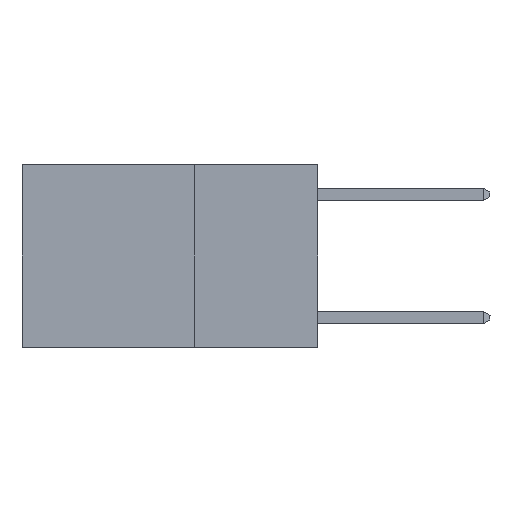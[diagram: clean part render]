
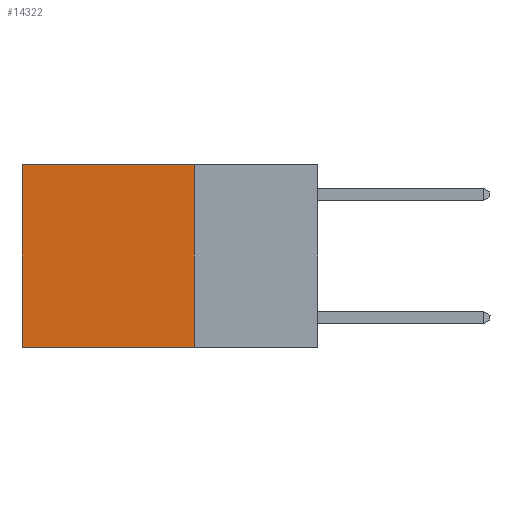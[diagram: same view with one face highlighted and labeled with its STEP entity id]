
A CAD part, left-side view. The second image highlights one B-rep face of the part: STEP entity #14322.
In plain terms, the highlighted planar face has unit normal (-1, 0, 0).
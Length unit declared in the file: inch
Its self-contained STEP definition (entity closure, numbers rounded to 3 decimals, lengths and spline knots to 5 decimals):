
#82 = PLANE ( 'NONE',  #14268 ) ;
#537 = LINE ( 'NONE', #14265, #15132 ) ;
#1487 = FACE_OUTER_BOUND ( 'NONE', #11805, .T. ) ;
#1881 = VERTEX_POINT ( 'NONE', #3082 ) ;
#2308 = VECTOR ( 'NONE', #5954, 39.37008 ) ;
#2724 = ORIENTED_EDGE ( 'NONE', *, *, #12147, .T. ) ;
#3082 = CARTESIAN_POINT ( 'NONE',  ( 0.2625, 0.6, 0. ) ) ;
#3145 = DIRECTION ( 'NONE',  ( 0., 1., 0. ) ) ;
#3184 = DIRECTION ( 'NONE',  ( 0., 0., -1. ) ) ;
#3637 = CARTESIAN_POINT ( 'NONE',  ( 0.2625, 0.25, -0.37 ) ) ;
#4820 = VERTEX_POINT ( 'NONE', #3637 ) ;
#4838 = VERTEX_POINT ( 'NONE', #14502 ) ;
#5202 = EDGE_CURVE ( 'NONE', #4820, #8546, #12601, .T. ) ;
#5829 = CARTESIAN_POINT ( 'NONE',  ( 0.2625, 0.25, -0.37 ) ) ;
#5954 = DIRECTION ( 'NONE',  ( 0., 0., -1. ) ) ;
#6131 = CARTESIAN_POINT ( 'NONE',  ( 0.2625, 0.6, 0. ) ) ;
#6523 = ORIENTED_EDGE ( 'NONE', *, *, #14434, .T. ) ;
#6581 = CARTESIAN_POINT ( 'NONE',  ( 0.2625, 0.25, 0. ) ) ;
#6945 = CARTESIAN_POINT ( 'NONE',  ( 0.2625, 0.25, 0. ) ) ;
#7928 = ORIENTED_EDGE ( 'NONE', *, *, #17227, .F. ) ;
#8546 = VERTEX_POINT ( 'NONE', #11970 ) ;
#9000 = LINE ( 'NONE', #6581, #17526 ) ;
#9831 = VECTOR ( 'NONE', #3145, 39.37008 ) ;
#9960 = LINE ( 'NONE', #6131, #2308 ) ;
#10339 = DIRECTION ( 'NONE',  ( 0., 0., -1. ) ) ;
#11805 = EDGE_LOOP ( 'NONE', ( #6523, #14726, #7928, #2724 ) ) ;
#11970 = CARTESIAN_POINT ( 'NONE',  ( 0.2625, 0.6, -0.37 ) ) ;
#12147 = EDGE_CURVE ( 'NONE', #4838, #1881, #537, .T. ) ;
#12601 = LINE ( 'NONE', #5829, #9831 ) ;
#13963 = DIRECTION ( 'NONE',  ( 1., 0., 0. ) ) ;
#14265 = CARTESIAN_POINT ( 'NONE',  ( 0.2625, 0.25, 0. ) ) ;
#14268 = AXIS2_PLACEMENT_3D ( 'NONE', #6945, #13963, #3184 ) ;
#14322 = ADVANCED_FACE ( 'NONE', ( #1487 ), #82, .F. ) ;
#14434 = EDGE_CURVE ( 'NONE', #1881, #8546, #9960, .T. ) ;
#14502 = CARTESIAN_POINT ( 'NONE',  ( 0.2625, 0.25, 0. ) ) ;
#14726 = ORIENTED_EDGE ( 'NONE', *, *, #5202, .F. ) ;
#15132 = VECTOR ( 'NONE', #15697, 39.37008 ) ;
#15697 = DIRECTION ( 'NONE',  ( 0., 1., 0. ) ) ;
#17227 = EDGE_CURVE ( 'NONE', #4838, #4820, #9000, .T. ) ;
#17526 = VECTOR ( 'NONE', #10339, 39.37008 ) ;
